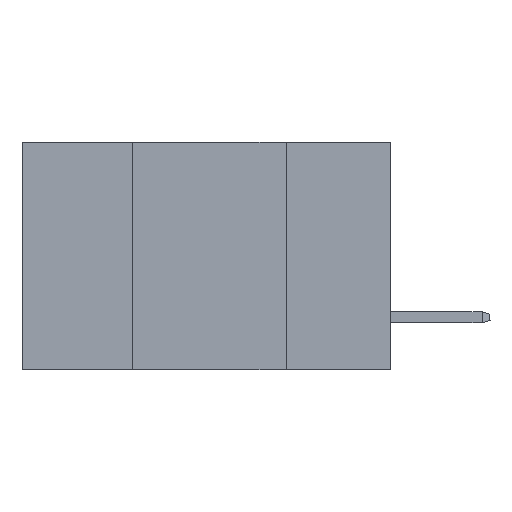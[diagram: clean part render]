
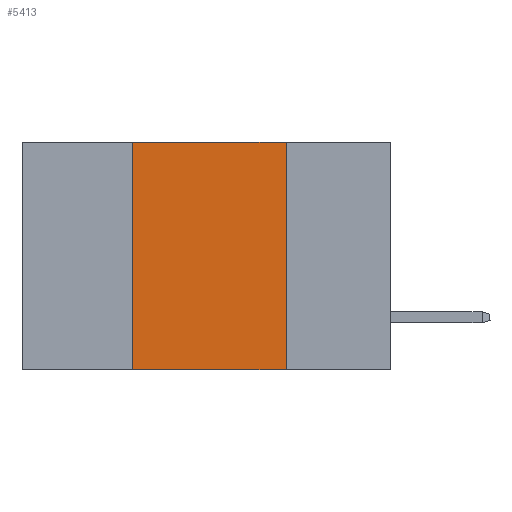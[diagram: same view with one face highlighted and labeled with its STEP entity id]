
A CAD part, left-side view. The second image highlights one B-rep face of the part: STEP entity #5413.
In plain terms, the highlighted planar face has unit normal (-1, 0, 0).
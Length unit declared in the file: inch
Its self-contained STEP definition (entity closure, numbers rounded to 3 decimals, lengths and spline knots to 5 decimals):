
#249 = ORIENTED_EDGE ( 'NONE', *, *, #13041, .F. ) ;
#807 = LINE ( 'NONE', #13068, #3904 ) ;
#1365 = CARTESIAN_POINT ( 'NONE',  ( 0., 0.42, -0.37 ) ) ;
#2733 = ORIENTED_EDGE ( 'NONE', *, *, #13756, .T. ) ;
#3425 = CARTESIAN_POINT ( 'NONE',  ( 0., 0.17, 0. ) ) ;
#3445 = FACE_OUTER_BOUND ( 'NONE', #6115, .T. ) ;
#3904 = VECTOR ( 'NONE', #4614, 39.37008 ) ;
#4614 = DIRECTION ( 'NONE',  ( 0., -1., 0. ) ) ;
#4850 = DIRECTION ( 'NONE',  ( 0., 0., -1. ) ) ;
#4939 = VERTEX_POINT ( 'NONE', #1365 ) ;
#5175 = ORIENTED_EDGE ( 'NONE', *, *, #15718, .F. ) ;
#5413 = ADVANCED_FACE ( 'NONE', ( #3445 ), #5507, .F. ) ;
#5507 = PLANE ( 'NONE',  #13181 ) ;
#6115 = EDGE_LOOP ( 'NONE', ( #9291, #249, #5175, #2733 ) ) ;
#6783 = LINE ( 'NONE', #16448, #15778 ) ;
#7808 = LINE ( 'NONE', #13679, #8007 ) ;
#8007 = VECTOR ( 'NONE', #10335, 39.37008 ) ;
#9136 = VECTOR ( 'NONE', #4850, 39.37008 ) ;
#9291 = ORIENTED_EDGE ( 'NONE', *, *, #14367, .F. ) ;
#9744 = CARTESIAN_POINT ( 'NONE',  ( 0., 0.6, 0. ) ) ;
#10335 = DIRECTION ( 'NONE',  ( 0., 0., 1. ) ) ;
#10477 = CARTESIAN_POINT ( 'NONE',  ( 0., 0.17, 0. ) ) ;
#10789 = DIRECTION ( 'NONE',  ( 0., -1., 0. ) ) ;
#13041 = EDGE_CURVE ( 'NONE', #13439, #13190, #6783, .T. ) ;
#13068 = CARTESIAN_POINT ( 'NONE',  ( 0., 0.6, -0.37 ) ) ;
#13181 = AXIS2_PLACEMENT_3D ( 'NONE', #9744, #16726, #18103 ) ;
#13190 = VERTEX_POINT ( 'NONE', #3425 ) ;
#13439 = VERTEX_POINT ( 'NONE', #16887 ) ;
#13679 = CARTESIAN_POINT ( 'NONE',  ( 0., 0.42, 0. ) ) ;
#13756 = EDGE_CURVE ( 'NONE', #4939, #16110, #807, .T. ) ;
#14367 = EDGE_CURVE ( 'NONE', #13190, #16110, #17940, .T. ) ;
#15641 = CARTESIAN_POINT ( 'NONE',  ( 0., 0.17, -0.37 ) ) ;
#15718 = EDGE_CURVE ( 'NONE', #4939, #13439, #7808, .T. ) ;
#15778 = VECTOR ( 'NONE', #10789, 39.37008 ) ;
#16110 = VERTEX_POINT ( 'NONE', #15641 ) ;
#16448 = CARTESIAN_POINT ( 'NONE',  ( 0., 0.6, 0. ) ) ;
#16726 = DIRECTION ( 'NONE',  ( 1., 0., 0. ) ) ;
#16887 = CARTESIAN_POINT ( 'NONE',  ( 0., 0.42, 0. ) ) ;
#17940 = LINE ( 'NONE', #10477, #9136 ) ;
#18103 = DIRECTION ( 'NONE',  ( 0., 0., -1. ) ) ;
